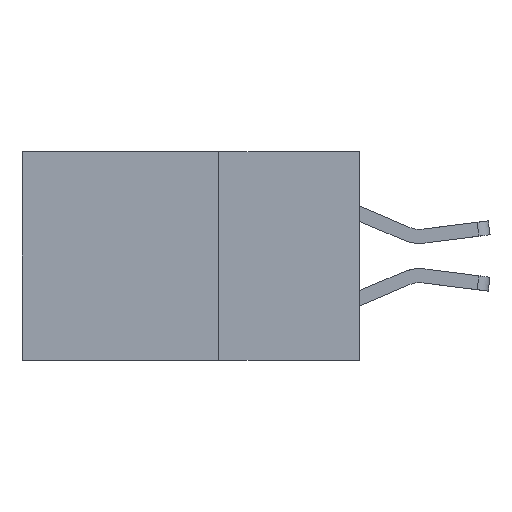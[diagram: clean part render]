
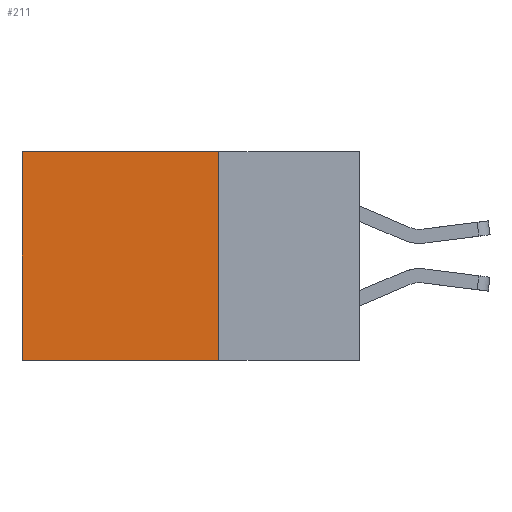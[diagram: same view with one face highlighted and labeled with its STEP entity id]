
A CAD part, left-side view. The second image highlights one B-rep face of the part: STEP entity #211.
In plain terms, the highlighted planar face has unit normal (-1, 0, 0).
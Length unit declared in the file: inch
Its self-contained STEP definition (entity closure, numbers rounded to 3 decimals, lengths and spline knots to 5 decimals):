
#90 = EDGE_CURVE ( 'NONE', #7729, #4671, #7516, .T. ) ;
#211 = ADVANCED_FACE ( 'NONE', ( #7837 ), #5773, .F. ) ;
#267 = CARTESIAN_POINT ( 'NONE',  ( 0.2875, 0.25, 0. ) ) ;
#485 = ORIENTED_EDGE ( 'NONE', *, *, #90, .T. ) ;
#1026 = LINE ( 'NONE', #7570, #2783 ) ;
#1184 = CARTESIAN_POINT ( 'NONE',  ( 0.2875, 0.6, 0. ) ) ;
#1404 = VERTEX_POINT ( 'NONE', #7099 ) ;
#1448 = ORIENTED_EDGE ( 'NONE', *, *, #2630, .F. ) ;
#1751 = ORIENTED_EDGE ( 'NONE', *, *, #8603, .F. ) ;
#2463 = ORIENTED_EDGE ( 'NONE', *, *, #2657, .T. ) ;
#2630 = EDGE_CURVE ( 'NONE', #1404, #7265, #7267, .T. ) ;
#2657 = EDGE_CURVE ( 'NONE', #4671, #7265, #7053, .T. ) ;
#2706 = DIRECTION ( 'NONE',  ( 0., 0., -1. ) ) ;
#2783 = VECTOR ( 'NONE', #5494, 39.37008 ) ;
#2806 = CARTESIAN_POINT ( 'NONE',  ( 0.2875, 0.25, 0. ) ) ;
#3353 = VECTOR ( 'NONE', #2706, 39.37008 ) ;
#3439 = DIRECTION ( 'NONE',  ( 0., 1., 0. ) ) ;
#3505 = CARTESIAN_POINT ( 'NONE',  ( 0.2875, 0.6, -0.37 ) ) ;
#3903 = DIRECTION ( 'NONE',  ( 1., 0., 0. ) ) ;
#4592 = DIRECTION ( 'NONE',  ( 0., 0., -1. ) ) ;
#4671 = VERTEX_POINT ( 'NONE', #1184 ) ;
#5352 = CARTESIAN_POINT ( 'NONE',  ( 0.2875, 0.25, -0.37 ) ) ;
#5431 = VECTOR ( 'NONE', #3439, 39.37008 ) ;
#5494 = DIRECTION ( 'NONE',  ( 0., 0., -1. ) ) ;
#5694 = VECTOR ( 'NONE', #8665, 39.37008 ) ;
#5773 = PLANE ( 'NONE',  #8144 ) ;
#5952 = CARTESIAN_POINT ( 'NONE',  ( 0.2875, 0.6, 0. ) ) ;
#7053 = LINE ( 'NONE', #5952, #3353 ) ;
#7099 = CARTESIAN_POINT ( 'NONE',  ( 0.2875, 0.25, -0.37 ) ) ;
#7265 = VERTEX_POINT ( 'NONE', #3505 ) ;
#7267 = LINE ( 'NONE', #5352, #5431 ) ;
#7516 = LINE ( 'NONE', #7918, #5694 ) ;
#7570 = CARTESIAN_POINT ( 'NONE',  ( 0.2875, 0.25, 0. ) ) ;
#7729 = VERTEX_POINT ( 'NONE', #267 ) ;
#7837 = FACE_OUTER_BOUND ( 'NONE', #8881, .T. ) ;
#7918 = CARTESIAN_POINT ( 'NONE',  ( 0.2875, 0.25, 0. ) ) ;
#8144 = AXIS2_PLACEMENT_3D ( 'NONE', #2806, #3903, #4592 ) ;
#8603 = EDGE_CURVE ( 'NONE', #7729, #1404, #1026, .T. ) ;
#8665 = DIRECTION ( 'NONE',  ( 0., 1., 0. ) ) ;
#8881 = EDGE_LOOP ( 'NONE', ( #2463, #1448, #1751, #485 ) ) ;
